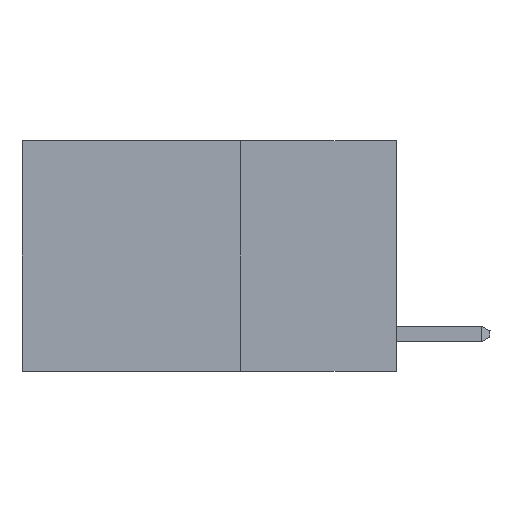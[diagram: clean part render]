
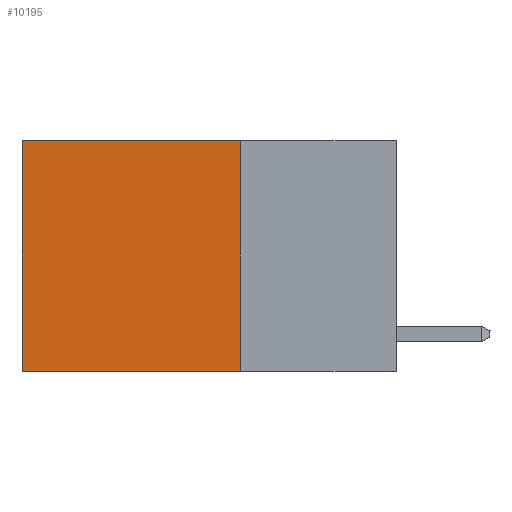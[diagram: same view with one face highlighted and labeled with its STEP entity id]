
A CAD part, left-side view. The second image highlights one B-rep face of the part: STEP entity #10195.
In plain terms, the highlighted planar face has unit normal (-1, 0, 0).
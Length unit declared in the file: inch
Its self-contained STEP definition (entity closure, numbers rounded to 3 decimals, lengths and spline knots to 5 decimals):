
#1588 = DIRECTION ( 'NONE',  ( 0., 0., -1. ) ) ;
#1792 = CARTESIAN_POINT ( 'NONE',  ( 0.2625, 0.25, 0. ) ) ;
#2361 = CARTESIAN_POINT ( 'NONE',  ( 0.2625, 0.25, 0. ) ) ;
#3218 = ORIENTED_EDGE ( 'NONE', *, *, #10938, .F. ) ;
#3396 = EDGE_LOOP ( 'NONE', ( #29709, #3218, #17398, #25967 ) ) ;
#6421 = VERTEX_POINT ( 'NONE', #28288 ) ;
#6810 = DIRECTION ( 'NONE',  ( 0., 0., -1. ) ) ;
#7484 = CARTESIAN_POINT ( 'NONE',  ( 0.2625, 0.25, -0.37 ) ) ;
#7909 = VECTOR ( 'NONE', #23269, 39.37008 ) ;
#8178 = CARTESIAN_POINT ( 'NONE',  ( 0.2625, 0.6, -0.37 ) ) ;
#8237 = LINE ( 'NONE', #7484, #26828 ) ;
#8893 = VERTEX_POINT ( 'NONE', #23558 ) ;
#9363 = CARTESIAN_POINT ( 'NONE',  ( 0.2625, 0.6, 0. ) ) ;
#10195 = ADVANCED_FACE ( 'NONE', ( #19717 ), #27821, .F. ) ;
#10850 = LINE ( 'NONE', #9363, #7909 ) ;
#10938 = EDGE_CURVE ( 'NONE', #6421, #11204, #8237, .T. ) ;
#11204 = VERTEX_POINT ( 'NONE', #8178 ) ;
#11290 = CARTESIAN_POINT ( 'NONE',  ( 0.2625, 0.25, 0. ) ) ;
#13237 = EDGE_CURVE ( 'NONE', #8893, #18161, #22960, .T. ) ;
#13719 = DIRECTION ( 'NONE',  ( 1., 0., 0. ) ) ;
#15487 = VECTOR ( 'NONE', #1588, 39.37008 ) ;
#17398 = ORIENTED_EDGE ( 'NONE', *, *, #26334, .F. ) ;
#18161 = VERTEX_POINT ( 'NONE', #22731 ) ;
#19717 = FACE_OUTER_BOUND ( 'NONE', #3396, .T. ) ;
#22731 = CARTESIAN_POINT ( 'NONE',  ( 0.2625, 0.6, 0. ) ) ;
#22849 = LINE ( 'NONE', #1792, #15487 ) ;
#22960 = LINE ( 'NONE', #2361, #28399 ) ;
#23132 = DIRECTION ( 'NONE',  ( 0., 1., 0. ) ) ;
#23269 = DIRECTION ( 'NONE',  ( 0., 0., -1. ) ) ;
#23486 = DIRECTION ( 'NONE',  ( 0., 1., 0. ) ) ;
#23558 = CARTESIAN_POINT ( 'NONE',  ( 0.2625, 0.25, 0. ) ) ;
#25223 = EDGE_CURVE ( 'NONE', #18161, #11204, #10850, .T. ) ;
#25967 = ORIENTED_EDGE ( 'NONE', *, *, #13237, .T. ) ;
#26334 = EDGE_CURVE ( 'NONE', #8893, #6421, #22849, .T. ) ;
#26828 = VECTOR ( 'NONE', #23132, 39.37008 ) ;
#27000 = AXIS2_PLACEMENT_3D ( 'NONE', #11290, #13719, #6810 ) ;
#27821 = PLANE ( 'NONE',  #27000 ) ;
#28288 = CARTESIAN_POINT ( 'NONE',  ( 0.2625, 0.25, -0.37 ) ) ;
#28399 = VECTOR ( 'NONE', #23486, 39.37008 ) ;
#29709 = ORIENTED_EDGE ( 'NONE', *, *, #25223, .T. ) ;
